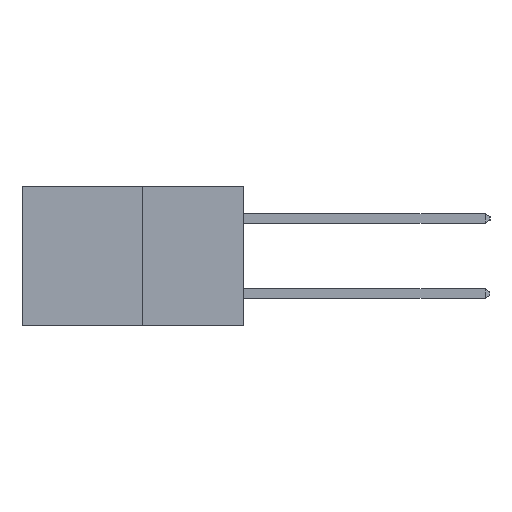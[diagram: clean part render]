
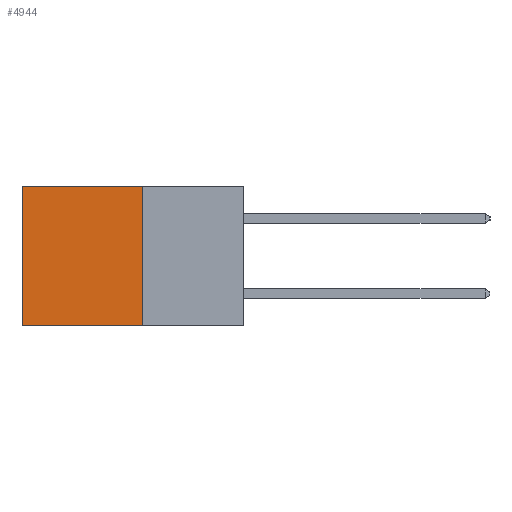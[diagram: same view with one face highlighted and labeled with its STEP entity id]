
A CAD part, left-side view. The second image highlights one B-rep face of the part: STEP entity #4944.
In plain terms, the highlighted planar face has unit normal (-1, 0, 0).
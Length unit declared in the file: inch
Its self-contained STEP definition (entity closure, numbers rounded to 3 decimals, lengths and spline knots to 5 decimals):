
#253 = LINE ( 'NONE', #8770, #2601 ) ;
#925 = VECTOR ( 'NONE', #12086, 39.37008 ) ;
#1186 = VERTEX_POINT ( 'NONE', #4422 ) ;
#1974 = CARTESIAN_POINT ( 'NONE',  ( 0.277, 0.27, -0.37 ) ) ;
#2002 = VECTOR ( 'NONE', #11701, 39.37008 ) ;
#2393 = AXIS2_PLACEMENT_3D ( 'NONE', #1974, #10835, #9981 ) ;
#2505 = CARTESIAN_POINT ( 'NONE',  ( 0.277, 0.59, -0.37 ) ) ;
#2601 = VECTOR ( 'NONE', #5761, 39.37008 ) ;
#3051 = EDGE_LOOP ( 'NONE', ( #9558, #11208, #10721, #11268 ) ) ;
#3272 = PLANE ( 'NONE',  #2393 ) ;
#3466 = CARTESIAN_POINT ( 'NONE',  ( 0.277, 0.27, -0.37 ) ) ;
#3529 = DIRECTION ( 'NONE',  ( 0., 0., -1. ) ) ;
#4422 = CARTESIAN_POINT ( 'NONE',  ( 0.277, 0.59, -0.37 ) ) ;
#4720 = VECTOR ( 'NONE', #3529, 39.37008 ) ;
#4944 = ADVANCED_FACE ( 'NONE', ( #7894 ), #3272, .F. ) ;
#5186 = CARTESIAN_POINT ( 'NONE',  ( 0.277, 0.27, -0.37 ) ) ;
#5761 = DIRECTION ( 'NONE',  ( 0., 1., 0. ) ) ;
#6183 = CARTESIAN_POINT ( 'NONE',  ( 0.277, 0.27, 0. ) ) ;
#6405 = VERTEX_POINT ( 'NONE', #6183 ) ;
#6707 = EDGE_CURVE ( 'NONE', #6405, #11842, #10021, .T. ) ;
#6897 = CARTESIAN_POINT ( 'NONE',  ( 0.277, 0.27, -0.37 ) ) ;
#7097 = LINE ( 'NONE', #6897, #2002 ) ;
#7833 = EDGE_CURVE ( 'NONE', #6405, #11594, #253, .T. ) ;
#7894 = FACE_OUTER_BOUND ( 'NONE', #3051, .T. ) ;
#8305 = LINE ( 'NONE', #2505, #925 ) ;
#8430 = EDGE_CURVE ( 'NONE', #11842, #1186, #7097, .T. ) ;
#8770 = CARTESIAN_POINT ( 'NONE',  ( 0.277, 0.27, 0. ) ) ;
#9558 = ORIENTED_EDGE ( 'NONE', *, *, #9770, .T. ) ;
#9770 = EDGE_CURVE ( 'NONE', #11594, #1186, #8305, .T. ) ;
#9981 = DIRECTION ( 'NONE',  ( 0., 0., -1. ) ) ;
#10021 = LINE ( 'NONE', #3466, #4720 ) ;
#10721 = ORIENTED_EDGE ( 'NONE', *, *, #6707, .F. ) ;
#10835 = DIRECTION ( 'NONE',  ( 1., 0., 0. ) ) ;
#10844 = CARTESIAN_POINT ( 'NONE',  ( 0.277, 0.59, 0. ) ) ;
#11208 = ORIENTED_EDGE ( 'NONE', *, *, #8430, .F. ) ;
#11268 = ORIENTED_EDGE ( 'NONE', *, *, #7833, .T. ) ;
#11594 = VERTEX_POINT ( 'NONE', #10844 ) ;
#11701 = DIRECTION ( 'NONE',  ( 0., 1., 0. ) ) ;
#11842 = VERTEX_POINT ( 'NONE', #5186 ) ;
#12086 = DIRECTION ( 'NONE',  ( 0., 0., -1. ) ) ;
